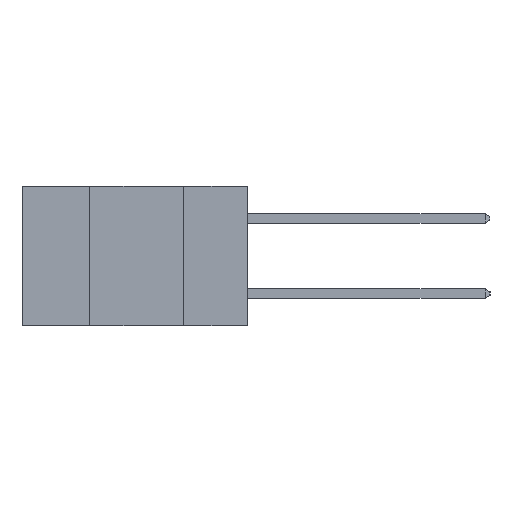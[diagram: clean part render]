
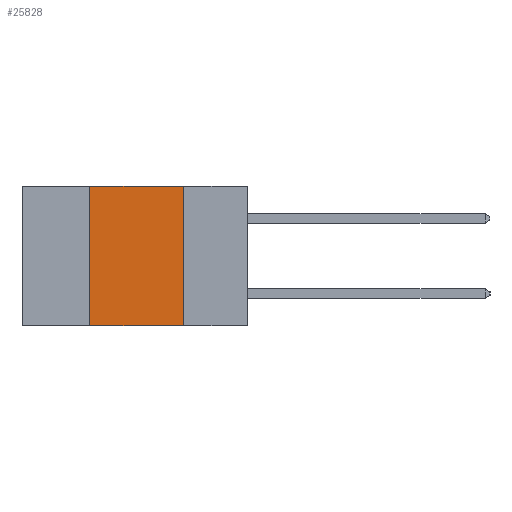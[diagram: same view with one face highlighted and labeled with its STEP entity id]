
A CAD part, left-side view. The second image highlights one B-rep face of the part: STEP entity #25828.
In plain terms, the highlighted planar face has unit normal (-1, 0, 0).
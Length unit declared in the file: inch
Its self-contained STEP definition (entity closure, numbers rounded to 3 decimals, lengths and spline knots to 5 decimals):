
#2921 = AXIS2_PLACEMENT_3D ( 'NONE', #12069, #16136, #3972 ) ;
#3123 = CARTESIAN_POINT ( 'NONE',  ( 0., 0.17, 0. ) ) ;
#3241 = CARTESIAN_POINT ( 'NONE',  ( 0., 0.42, 0. ) ) ;
#3404 = VECTOR ( 'NONE', #3462, 39.37008 ) ;
#3462 = DIRECTION ( 'NONE',  ( 0., -1., 0. ) ) ;
#3972 = DIRECTION ( 'NONE',  ( 0., 0., -1. ) ) ;
#4477 = LINE ( 'NONE', #5541, #20019 ) ;
#5541 = CARTESIAN_POINT ( 'NONE',  ( 0., 0.6, -0.37 ) ) ;
#6407 = ORIENTED_EDGE ( 'NONE', *, *, #10759, .F. ) ;
#7032 = ORIENTED_EDGE ( 'NONE', *, *, #8064, .T. ) ;
#7638 = DIRECTION ( 'NONE',  ( 0., 0., -1. ) ) ;
#7862 = VECTOR ( 'NONE', #7638, 39.37008 ) ;
#7984 = PLANE ( 'NONE',  #2921 ) ;
#8064 = EDGE_CURVE ( 'NONE', #15895, #20082, #4477, .T. ) ;
#8482 = LINE ( 'NONE', #23669, #7862 ) ;
#8608 = FACE_OUTER_BOUND ( 'NONE', #16277, .T. ) ;
#9388 = VERTEX_POINT ( 'NONE', #3241 ) ;
#9420 = EDGE_CURVE ( 'NONE', #15895, #9388, #19945, .T. ) ;
#10759 = EDGE_CURVE ( 'NONE', #9388, #11898, #18946, .T. ) ;
#11898 = VERTEX_POINT ( 'NONE', #3123 ) ;
#12069 = CARTESIAN_POINT ( 'NONE',  ( 0., 0.6, 0. ) ) ;
#13469 = CARTESIAN_POINT ( 'NONE',  ( 0., 0.42, -0.37 ) ) ;
#14586 = VECTOR ( 'NONE', #21504, 39.37008 ) ;
#15895 = VERTEX_POINT ( 'NONE', #25304 ) ;
#16136 = DIRECTION ( 'NONE',  ( 1., 0., 0. ) ) ;
#16277 = EDGE_LOOP ( 'NONE', ( #16569, #6407, #22524, #7032 ) ) ;
#16569 = ORIENTED_EDGE ( 'NONE', *, *, #17547, .F. ) ;
#17547 = EDGE_CURVE ( 'NONE', #11898, #20082, #8482, .T. ) ;
#18946 = LINE ( 'NONE', #19681, #3404 ) ;
#19681 = CARTESIAN_POINT ( 'NONE',  ( 0., 0.6, 0. ) ) ;
#19709 = DIRECTION ( 'NONE',  ( 0., -1., 0. ) ) ;
#19945 = LINE ( 'NONE', #13469, #14586 ) ;
#20019 = VECTOR ( 'NONE', #19709, 39.37008 ) ;
#20082 = VERTEX_POINT ( 'NONE', #25540 ) ;
#21504 = DIRECTION ( 'NONE',  ( 0., 0., 1. ) ) ;
#22524 = ORIENTED_EDGE ( 'NONE', *, *, #9420, .F. ) ;
#23669 = CARTESIAN_POINT ( 'NONE',  ( 0., 0.17, -0.37 ) ) ;
#25304 = CARTESIAN_POINT ( 'NONE',  ( 0., 0.42, -0.37 ) ) ;
#25540 = CARTESIAN_POINT ( 'NONE',  ( 0., 0.17, -0.37 ) ) ;
#25828 = ADVANCED_FACE ( 'NONE', ( #8608 ), #7984, .F. ) ;
